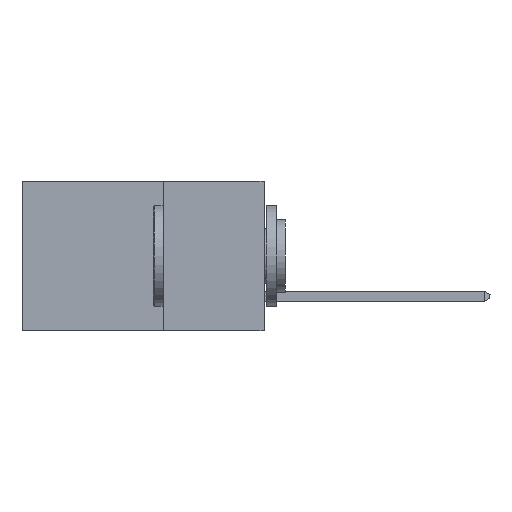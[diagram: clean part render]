
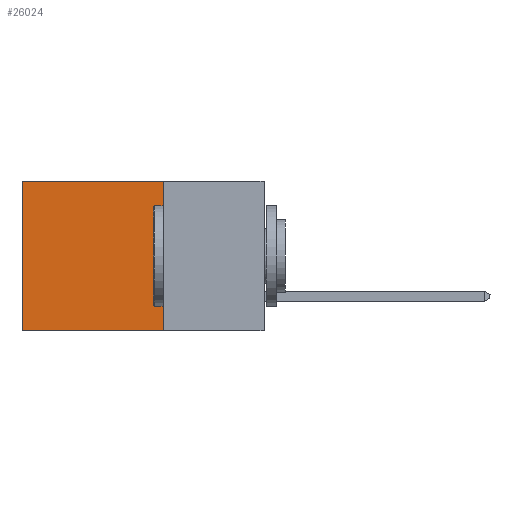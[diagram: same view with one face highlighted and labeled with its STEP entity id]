
A CAD part, left-side view. The second image highlights one B-rep face of the part: STEP entity #26024.
In plain terms, the highlighted planar face has unit normal (-1, 0, 0).
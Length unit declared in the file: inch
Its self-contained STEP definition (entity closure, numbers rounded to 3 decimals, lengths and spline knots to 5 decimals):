
#427 = LINE ( 'NONE', #24454, #23883 ) ;
#555 = DIRECTION ( 'NONE',  ( 1., 0., 0. ) ) ;
#739 = VERTEX_POINT ( 'NONE', #19064 ) ;
#1416 = DIRECTION ( 'NONE',  ( 0., 1., 0. ) ) ;
#4131 = CARTESIAN_POINT ( 'NONE',  ( 0.298, 0.6, 0. ) ) ;
#5449 = LINE ( 'NONE', #27918, #28585 ) ;
#6574 = EDGE_LOOP ( 'NONE', ( #19657, #6915, #14847, #21133 ) ) ;
#6915 = ORIENTED_EDGE ( 'NONE', *, *, #14656, .F. ) ;
#8628 = VERTEX_POINT ( 'NONE', #22389 ) ;
#9019 = CARTESIAN_POINT ( 'NONE',  ( 0.298, 0.6, 0. ) ) ;
#9805 = DIRECTION ( 'NONE',  ( 0., 0., -1. ) ) ;
#11128 = VECTOR ( 'NONE', #1416, 39.37008 ) ;
#11210 = EDGE_CURVE ( 'NONE', #8628, #11773, #427, .T. ) ;
#11773 = VERTEX_POINT ( 'NONE', #9019 ) ;
#14284 = PLANE ( 'NONE',  #20436 ) ;
#14656 = EDGE_CURVE ( 'NONE', #18854, #739, #26471, .T. ) ;
#14847 = ORIENTED_EDGE ( 'NONE', *, *, #24799, .F. ) ;
#15503 = EDGE_CURVE ( 'NONE', #11773, #739, #16770, .T. ) ;
#16770 = LINE ( 'NONE', #4131, #27455 ) ;
#18831 = CARTESIAN_POINT ( 'NONE',  ( 0.298, 0.25, 0. ) ) ;
#18854 = VERTEX_POINT ( 'NONE', #25493 ) ;
#19064 = CARTESIAN_POINT ( 'NONE',  ( 0.298, 0.6, -0.37 ) ) ;
#19657 = ORIENTED_EDGE ( 'NONE', *, *, #15503, .T. ) ;
#20436 = AXIS2_PLACEMENT_3D ( 'NONE', #18831, #555, #25730 ) ;
#21133 = ORIENTED_EDGE ( 'NONE', *, *, #11210, .T. ) ;
#22104 = FACE_OUTER_BOUND ( 'NONE', #6574, .T. ) ;
#22389 = CARTESIAN_POINT ( 'NONE',  ( 0.298, 0.25, 0. ) ) ;
#22467 = CARTESIAN_POINT ( 'NONE',  ( 0.298, 0.25, -0.37 ) ) ;
#23883 = VECTOR ( 'NONE', #24345, 39.37008 ) ;
#24345 = DIRECTION ( 'NONE',  ( 0., 1., 0. ) ) ;
#24454 = CARTESIAN_POINT ( 'NONE',  ( 0.298, 0.25, 0. ) ) ;
#24799 = EDGE_CURVE ( 'NONE', #8628, #18854, #5449, .T. ) ;
#25493 = CARTESIAN_POINT ( 'NONE',  ( 0.298, 0.25, -0.37 ) ) ;
#25730 = DIRECTION ( 'NONE',  ( 0., 0., -1. ) ) ;
#26024 = ADVANCED_FACE ( 'NONE', ( #22104 ), #14284, .F. ) ;
#26471 = LINE ( 'NONE', #22467, #11128 ) ;
#27455 = VECTOR ( 'NONE', #29184, 39.37008 ) ;
#27918 = CARTESIAN_POINT ( 'NONE',  ( 0.298, 0.25, 0. ) ) ;
#28585 = VECTOR ( 'NONE', #9805, 39.37008 ) ;
#29184 = DIRECTION ( 'NONE',  ( 0., 0., -1. ) ) ;
